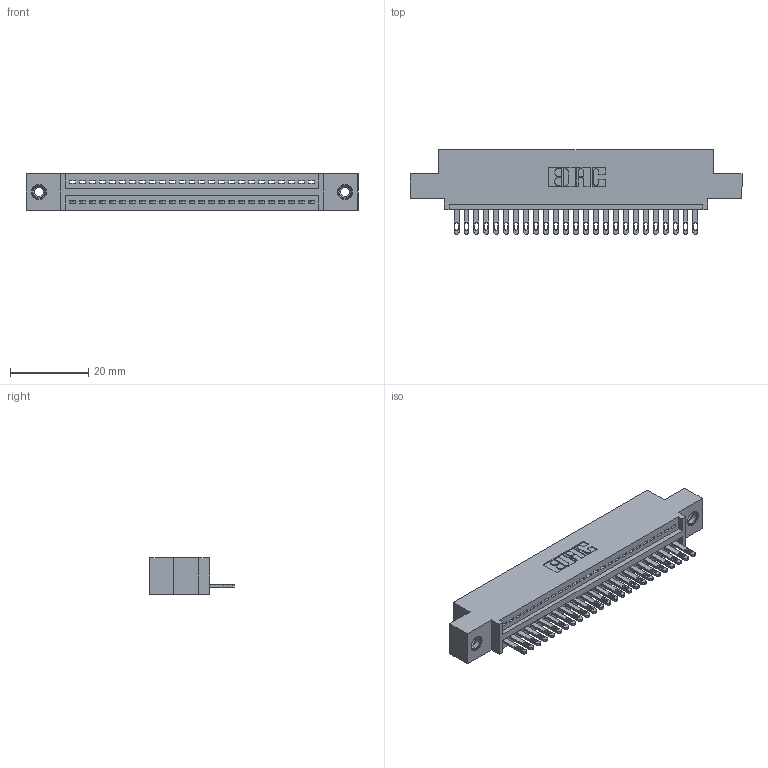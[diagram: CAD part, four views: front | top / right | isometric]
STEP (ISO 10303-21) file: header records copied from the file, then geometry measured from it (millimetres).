
FILE_DESCRIPTION (( 'STEP AP203' ), '1' );
FILE_NAME ('345-025-500-408.STEP', '2019-10-05T05:45:32', ( '' ), ( '' ), 'SwSTEP 2.0', 'SolidWorks 2016', '' );
FILE_SCHEMA (( 'CONFIG_CONTROL_DESIGN' ));
Length unit declared in the file: inch
Products named in the file (4): 345-025-500-408; 345-292-001_345-293-100; 345-250-001_345-250-003-102; 345 Part_0.110 Offset - 0.156 Dia-TI
Assembly tree (28 placements, depth 2):
  345-025-500-408
    345 Part_0.110 Offset - 0.156 Dia-TI
    345-292-001_345-293-100  x25
    345-250-001_345-250-003-102  x2
Bounding box: 84.71 x 21.51 x 9.4 mm (x, y, z)
Volume: 7842.1 mm3; surface area: 10347.5 mm2
Topology: 28 solids, 28 shells, 1540 faces, 4689 edges, 3118 vertices
Faces by surface type: plane 966, cylinder 558, cone 12, torus 4
Entity records: 22352 total; most frequent: CARTESIAN_POINT 3854, ORIENTED_EDGE 3806, DIRECTION 3419, EDGE_CURVE 1903, LINE 1647, VECTOR 1647, VERTEX_POINT 1264, AXIS2_PLACEMENT_3D 886
